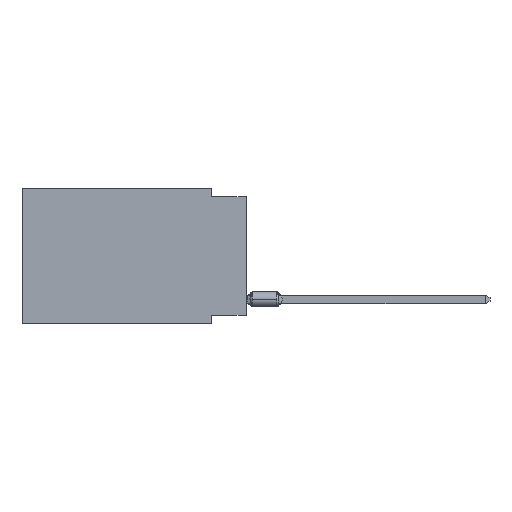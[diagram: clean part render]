
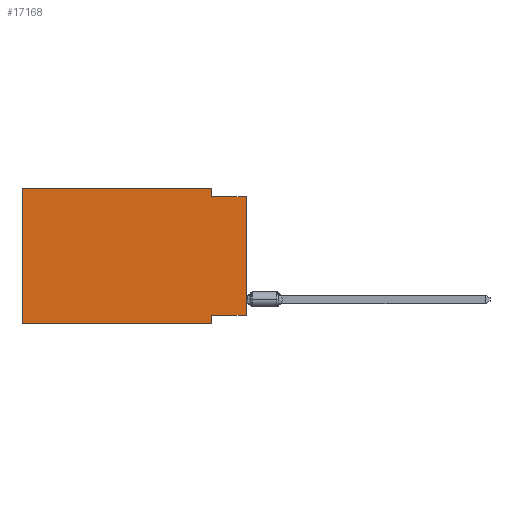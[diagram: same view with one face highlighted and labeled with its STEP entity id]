
A CAD part, left-side view. The second image highlights one B-rep face of the part: STEP entity #17168.
In plain terms, the highlighted planar face has unit normal (-1, 0, 0).
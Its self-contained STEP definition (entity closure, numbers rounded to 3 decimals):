
#165 = ORIENTED_EDGE ( 'NONE', *, *, #8567, .T. ) ;
#704 = CARTESIAN_POINT ( 'NONE',  ( 0., 2.54, -0.635 ) ) ;
#748 = DIRECTION ( 'NONE',  ( 1., 0., 0. ) ) ;
#892 = LINE ( 'NONE', #17756, #16719 ) ;
#1018 = VERTEX_POINT ( 'NONE', #15989 ) ;
#1073 = DIRECTION ( 'NONE',  ( 0., 0., -1. ) ) ;
#1413 = LINE ( 'NONE', #20216, #10435 ) ;
#1706 = CARTESIAN_POINT ( 'NONE',  ( 0., 16.383, -9.906 ) ) ;
#2255 = VERTEX_POINT ( 'NONE', #704 ) ;
#2267 = EDGE_CURVE ( 'NONE', #11977, #13198, #4302, .T. ) ;
#2478 = LINE ( 'NONE', #5752, #13940 ) ;
#2637 = ORIENTED_EDGE ( 'NONE', *, *, #12002, .F. ) ;
#2815 = EDGE_CURVE ( 'NONE', #2255, #1018, #18906, .T. ) ;
#3160 = DIRECTION ( 'NONE',  ( 0., -1., 0. ) ) ;
#3440 = VERTEX_POINT ( 'NONE', #5364 ) ;
#3480 = CARTESIAN_POINT ( 'NONE',  ( 0., 2.54, -9.906 ) ) ;
#3707 = DIRECTION ( 'NONE',  ( 0., 0., 1. ) ) ;
#4107 = ORIENTED_EDGE ( 'NONE', *, *, #11755, .F. ) ;
#4163 = VECTOR ( 'NONE', #12947, 1000. ) ;
#4302 = LINE ( 'NONE', #21411, #4163 ) ;
#5364 = CARTESIAN_POINT ( 'NONE',  ( 0., 2.54, -9.271 ) ) ;
#5557 = VECTOR ( 'NONE', #12937, 1000. ) ;
#5752 = CARTESIAN_POINT ( 'NONE',  ( 0., 16.383, 0. ) ) ;
#5867 = CARTESIAN_POINT ( 'NONE',  ( 0., 2.54, 0. ) ) ;
#5946 = FACE_OUTER_BOUND ( 'NONE', #13697, .T. ) ;
#6390 = VERTEX_POINT ( 'NONE', #8540 ) ;
#7324 = DIRECTION ( 'NONE',  ( 0., 0., -1. ) ) ;
#7579 = CARTESIAN_POINT ( 'NONE',  ( 0., 2.54, 0. ) ) ;
#7631 = PLANE ( 'NONE',  #19003 ) ;
#8030 = DIRECTION ( 'NONE',  ( 0., 1., 0. ) ) ;
#8308 = DIRECTION ( 'NONE',  ( 0., -1., 0. ) ) ;
#8480 = CARTESIAN_POINT ( 'NONE',  ( 0., 0., -0.635 ) ) ;
#8540 = CARTESIAN_POINT ( 'NONE',  ( 0., 0., -9.271 ) ) ;
#8567 = EDGE_CURVE ( 'NONE', #6390, #1018, #12330, .T. ) ;
#9411 = ORIENTED_EDGE ( 'NONE', *, *, #10442, .F. ) ;
#9695 = CARTESIAN_POINT ( 'NONE',  ( 0., 16.383, 0. ) ) ;
#10049 = ORIENTED_EDGE ( 'NONE', *, *, #18321, .F. ) ;
#10435 = VECTOR ( 'NONE', #8308, 1000. ) ;
#10442 = EDGE_CURVE ( 'NONE', #10854, #2255, #18124, .T. ) ;
#10550 = VECTOR ( 'NONE', #3160, 1000. ) ;
#10854 = VERTEX_POINT ( 'NONE', #5867 ) ;
#11071 = VERTEX_POINT ( 'NONE', #19111 ) ;
#11397 = VECTOR ( 'NONE', #3707, 1000. ) ;
#11603 = ORIENTED_EDGE ( 'NONE', *, *, #2267, .T. ) ;
#11755 = EDGE_CURVE ( 'NONE', #6390, #3440, #13151, .T. ) ;
#11977 = VERTEX_POINT ( 'NONE', #1706 ) ;
#12002 = EDGE_CURVE ( 'NONE', #11977, #11071, #2478, .T. ) ;
#12330 = LINE ( 'NONE', #19235, #11397 ) ;
#12937 = DIRECTION ( 'NONE',  ( 0., 0., -1. ) ) ;
#12947 = DIRECTION ( 'NONE',  ( 0., -1., 0. ) ) ;
#13151 = LINE ( 'NONE', #17107, #15386 ) ;
#13198 = VERTEX_POINT ( 'NONE', #3480 ) ;
#13697 = EDGE_LOOP ( 'NONE', ( #165, #21140, #9411, #16750, #2637, #11603, #10049, #4107 ) ) ;
#13940 = VECTOR ( 'NONE', #19467, 1000. ) ;
#15166 = EDGE_CURVE ( 'NONE', #11071, #10854, #1413, .T. ) ;
#15386 = VECTOR ( 'NONE', #8030, 1000. ) ;
#15989 = CARTESIAN_POINT ( 'NONE',  ( 0., 0., -0.635 ) ) ;
#16719 = VECTOR ( 'NONE', #7324, 1000. ) ;
#16750 = ORIENTED_EDGE ( 'NONE', *, *, #15166, .F. ) ;
#17107 = CARTESIAN_POINT ( 'NONE',  ( 0., 0., -9.271 ) ) ;
#17168 = ADVANCED_FACE ( 'NONE', ( #5946 ), #7631, .F. ) ;
#17756 = CARTESIAN_POINT ( 'NONE',  ( 0., 2.54, -9.906 ) ) ;
#18124 = LINE ( 'NONE', #7579, #5557 ) ;
#18321 = EDGE_CURVE ( 'NONE', #3440, #13198, #892, .T. ) ;
#18906 = LINE ( 'NONE', #8480, #10550 ) ;
#19003 = AXIS2_PLACEMENT_3D ( 'NONE', #9695, #748, #1073 ) ;
#19111 = CARTESIAN_POINT ( 'NONE',  ( 0., 16.383, 0. ) ) ;
#19235 = CARTESIAN_POINT ( 'NONE',  ( 0., 0., 0. ) ) ;
#19467 = DIRECTION ( 'NONE',  ( 0., 0., 1. ) ) ;
#20216 = CARTESIAN_POINT ( 'NONE',  ( 0., 16.383, 0. ) ) ;
#21140 = ORIENTED_EDGE ( 'NONE', *, *, #2815, .F. ) ;
#21411 = CARTESIAN_POINT ( 'NONE',  ( 0., 16.383, -9.906 ) ) ;
